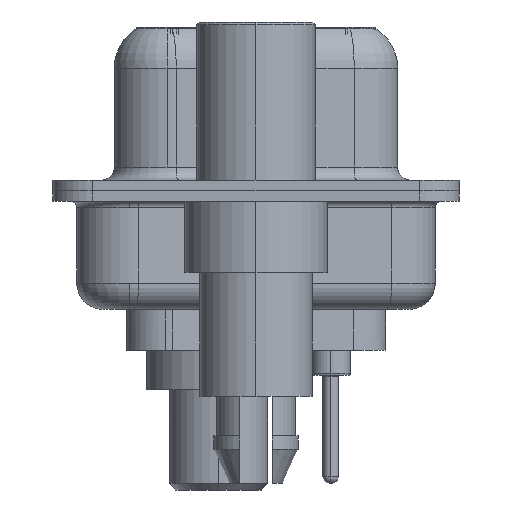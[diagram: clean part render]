
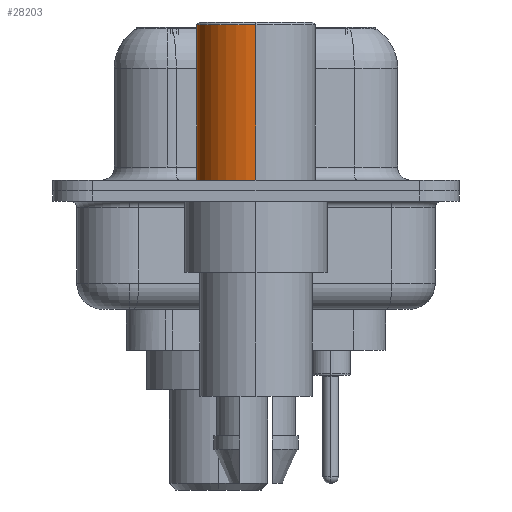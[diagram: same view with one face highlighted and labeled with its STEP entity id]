
A CAD part, left-side view. The second image highlights one B-rep face of the part: STEP entity #28203.
In plain terms, the highlighted cylindrical face has radius 2.25 mm (diameter 4.5 mm), a partial arc.
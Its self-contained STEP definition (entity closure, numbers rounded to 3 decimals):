
#171 = CARTESIAN_POINT ( 'NONE',  ( 2.25, 0., 0.581 ) ) ;
#1233 = VERTEX_POINT ( 'NONE', #20939 ) ;
#1554 = ORIENTED_EDGE ( 'NONE', *, *, #30163, .F. ) ;
#1796 = FACE_OUTER_BOUND ( 'NONE', #24888, .T. ) ;
#1955 = DIRECTION ( 'NONE',  ( 1., 0., 0. ) ) ;
#2709 = VECTOR ( 'NONE', #9455, 1000. ) ;
#3931 = CARTESIAN_POINT ( 'NONE',  ( 0., 0., 0.4 ) ) ;
#6197 = EDGE_CURVE ( 'NONE', #30401, #1233, #19564, .T. ) ;
#8207 = VERTEX_POINT ( 'NONE', #31092 ) ;
#9446 = LINE ( 'NONE', #14230, #2709 ) ;
#9455 = DIRECTION ( 'NONE',  ( 0., 0., 1. ) ) ;
#10173 = ORIENTED_EDGE ( 'NONE', *, *, #14492, .T. ) ;
#10195 = DIRECTION ( 'NONE',  ( 0., 0., 1. ) ) ;
#11801 = CIRCLE ( 'NONE', #15813, 2.25 ) ;
#12246 = CARTESIAN_POINT ( 'NONE',  ( 0., 0., 0.581 ) ) ;
#14230 = CARTESIAN_POINT ( 'NONE',  ( -2.25, 0., 0.581 ) ) ;
#14451 = CIRCLE ( 'NONE', #25387, 2.25 ) ;
#14492 = EDGE_CURVE ( 'NONE', #30401, #24897, #11801, .T. ) ;
#14578 = EDGE_CURVE ( 'NONE', #24897, #8207, #9446, .T. ) ;
#14846 = DIRECTION ( 'NONE',  ( 1., 0., 0. ) ) ;
#15813 = AXIS2_PLACEMENT_3D ( 'NONE', #3931, #16360, #19115 ) ;
#15830 = ORIENTED_EDGE ( 'NONE', *, *, #14578, .T. ) ;
#16360 = DIRECTION ( 'NONE',  ( 0., 0., 1. ) ) ;
#17122 = CARTESIAN_POINT ( 'NONE',  ( 0., 0., 6.3 ) ) ;
#19115 = DIRECTION ( 'NONE',  ( 1., 0., 0. ) ) ;
#19564 = LINE ( 'NONE', #171, #27754 ) ;
#20939 = CARTESIAN_POINT ( 'NONE',  ( 2.25, 0., 6.3 ) ) ;
#21800 = ORIENTED_EDGE ( 'NONE', *, *, #6197, .F. ) ;
#22156 = AXIS2_PLACEMENT_3D ( 'NONE', #12246, #29837, #14846 ) ;
#24677 = CARTESIAN_POINT ( 'NONE',  ( -2.25, 0., 0.4 ) ) ;
#24888 = EDGE_LOOP ( 'NONE', ( #10173, #15830, #1554, #21800 ) ) ;
#24897 = VERTEX_POINT ( 'NONE', #24677 ) ;
#25387 = AXIS2_PLACEMENT_3D ( 'NONE', #17122, #31796, #1955 ) ;
#25434 = CYLINDRICAL_SURFACE ( 'NONE', #22156, 2.25 ) ;
#27754 = VECTOR ( 'NONE', #10195, 1000. ) ;
#28140 = CARTESIAN_POINT ( 'NONE',  ( 2.25, 0., 0.4 ) ) ;
#28203 = ADVANCED_FACE ( 'NONE', ( #1796 ), #25434, .T. ) ;
#29837 = DIRECTION ( 'NONE',  ( 0., 0., 1. ) ) ;
#30163 = EDGE_CURVE ( 'NONE', #1233, #8207, #14451, .T. ) ;
#30401 = VERTEX_POINT ( 'NONE', #28140 ) ;
#31092 = CARTESIAN_POINT ( 'NONE',  ( -2.25, 0., 6.3 ) ) ;
#31796 = DIRECTION ( 'NONE',  ( 0., 0., 1. ) ) ;
